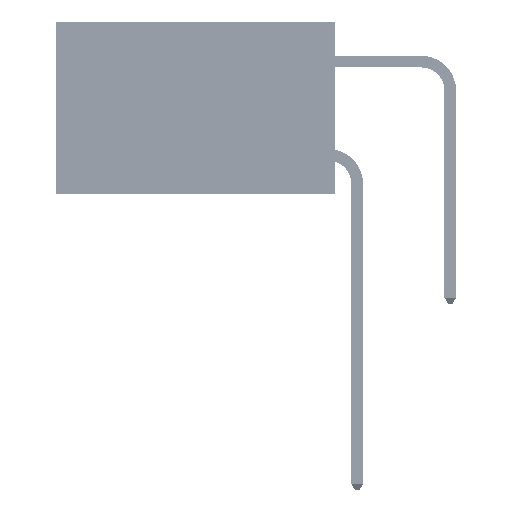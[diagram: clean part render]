
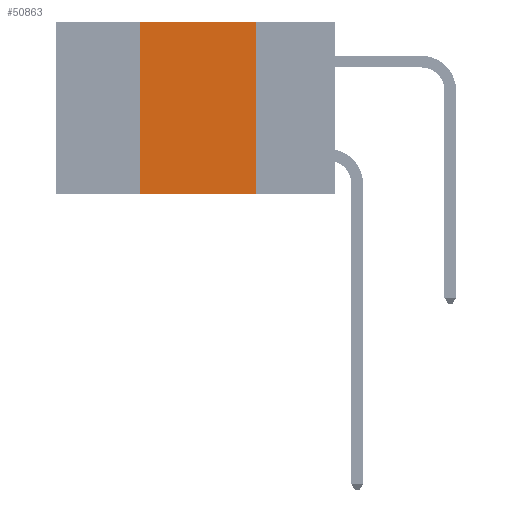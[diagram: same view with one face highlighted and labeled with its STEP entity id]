
A CAD part, left-side view. The second image highlights one B-rep face of the part: STEP entity #50863.
In plain terms, the highlighted planar face has unit normal (-1, 0, 0).
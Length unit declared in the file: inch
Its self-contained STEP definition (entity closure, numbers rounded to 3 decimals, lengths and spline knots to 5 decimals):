
#548 = ORIENTED_EDGE ( 'NONE', *, *, #35944, .F. ) ;
#1554 = CARTESIAN_POINT ( 'NONE',  ( 0., 0.17, -0.37 ) ) ;
#4136 = CARTESIAN_POINT ( 'NONE',  ( 0., 0.17, 0. ) ) ;
#7459 = VERTEX_POINT ( 'NONE', #54000 ) ;
#9926 = VERTEX_POINT ( 'NONE', #1554 ) ;
#10894 = EDGE_CURVE ( 'NONE', #21811, #14584, #13504, .T. ) ;
#13299 = DIRECTION ( 'NONE',  ( 1., 0., 0. ) ) ;
#13504 = LINE ( 'NONE', #43032, #24821 ) ;
#14584 = VERTEX_POINT ( 'NONE', #45249 ) ;
#14667 = VECTOR ( 'NONE', #20846, 39.37008 ) ;
#18888 = ORIENTED_EDGE ( 'NONE', *, *, #10894, .F. ) ;
#19115 = VECTOR ( 'NONE', #52732, 39.37008 ) ;
#20846 = DIRECTION ( 'NONE',  ( 0., 0., -1. ) ) ;
#20959 = DIRECTION ( 'NONE',  ( 0., 0., -1. ) ) ;
#21154 = EDGE_LOOP ( 'NONE', ( #21209, #548, #18888, #50857 ) ) ;
#21209 = ORIENTED_EDGE ( 'NONE', *, *, #46777, .F. ) ;
#21811 = VERTEX_POINT ( 'NONE', #36842 ) ;
#24821 = VECTOR ( 'NONE', #26062, 39.37008 ) ;
#25594 = CARTESIAN_POINT ( 'NONE',  ( 0., 0.6, 0. ) ) ;
#26062 = DIRECTION ( 'NONE',  ( 0., 0., 1. ) ) ;
#29173 = DIRECTION ( 'NONE',  ( 0., -1., 0. ) ) ;
#34320 = FACE_OUTER_BOUND ( 'NONE', #21154, .T. ) ;
#35944 = EDGE_CURVE ( 'NONE', #14584, #7459, #40149, .T. ) ;
#36842 = CARTESIAN_POINT ( 'NONE',  ( 0., 0.42, -0.37 ) ) ;
#38199 = LINE ( 'NONE', #46431, #42641 ) ;
#38702 = PLANE ( 'NONE',  #40162 ) ;
#40149 = LINE ( 'NONE', #48645, #19115 ) ;
#40162 = AXIS2_PLACEMENT_3D ( 'NONE', #25594, #13299, #20959 ) ;
#41614 = LINE ( 'NONE', #4136, #14667 ) ;
#42641 = VECTOR ( 'NONE', #29173, 39.37008 ) ;
#43032 = CARTESIAN_POINT ( 'NONE',  ( 0., 0.42, 0. ) ) ;
#45249 = CARTESIAN_POINT ( 'NONE',  ( 0., 0.42, 0. ) ) ;
#46431 = CARTESIAN_POINT ( 'NONE',  ( 0., 0.6, -0.37 ) ) ;
#46777 = EDGE_CURVE ( 'NONE', #7459, #9926, #41614, .T. ) ;
#48645 = CARTESIAN_POINT ( 'NONE',  ( 0., 0.6, 0. ) ) ;
#48836 = EDGE_CURVE ( 'NONE', #21811, #9926, #38199, .T. ) ;
#50857 = ORIENTED_EDGE ( 'NONE', *, *, #48836, .T. ) ;
#50863 = ADVANCED_FACE ( 'NONE', ( #34320 ), #38702, .F. ) ;
#52732 = DIRECTION ( 'NONE',  ( 0., -1., 0. ) ) ;
#54000 = CARTESIAN_POINT ( 'NONE',  ( 0., 0.17, 0. ) ) ;
